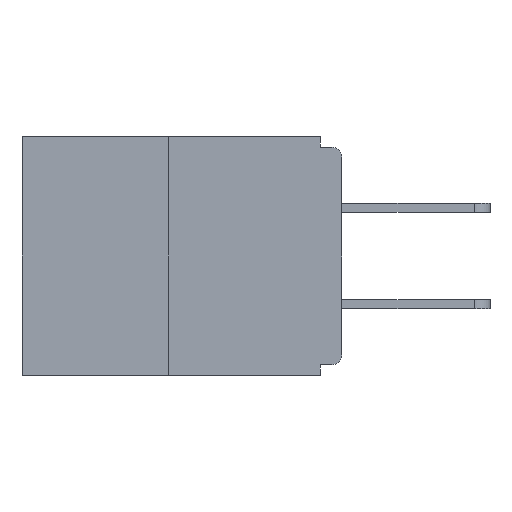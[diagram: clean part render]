
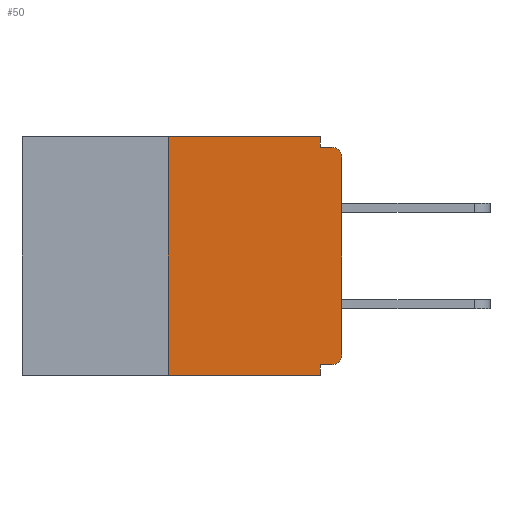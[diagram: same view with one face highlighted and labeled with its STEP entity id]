
A CAD part, left-side view. The second image highlights one B-rep face of the part: STEP entity #50.
In plain terms, the highlighted planar face has unit normal (-1, 0, 0).
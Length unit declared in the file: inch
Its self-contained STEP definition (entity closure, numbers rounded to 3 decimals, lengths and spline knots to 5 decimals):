
#50 = ADVANCED_FACE ( 'NONE', ( #7094 ), #10896, .F. ) ;
#77 = CARTESIAN_POINT ( 'NONE',  ( 0., 0.46, 0. ) ) ;
#176 = VECTOR ( 'NONE', #2043, 39.37008 ) ;
#850 = CARTESIAN_POINT ( 'NONE',  ( 0., 0., -0.313 ) ) ;
#913 = VERTEX_POINT ( 'NONE', #2704 ) ;
#1152 = ORIENTED_EDGE ( 'NONE', *, *, #24956, .F. ) ;
#1242 = EDGE_CURVE ( 'NONE', #12072, #3037, #13367, .T. ) ;
#1349 = VECTOR ( 'NONE', #26919, 39.37008 ) ;
#1949 = DIRECTION ( 'NONE',  ( 0., 0., -1. ) ) ;
#2043 = DIRECTION ( 'NONE',  ( 0., 0., 1. ) ) ;
#2326 = DIRECTION ( 'NONE',  ( 0., 0., -1. ) ) ;
#2608 = CARTESIAN_POINT ( 'NONE',  ( 0., 0.015, -0.015 ) ) ;
#2704 = CARTESIAN_POINT ( 'NONE',  ( 0., 0.25, 0. ) ) ;
#3037 = VERTEX_POINT ( 'NONE', #6431 ) ;
#3648 = CARTESIAN_POINT ( 'NONE',  ( 0., 0.031, -0.343 ) ) ;
#4474 = AXIS2_PLACEMENT_3D ( 'NONE', #77, #15582, #1949 ) ;
#4501 = DIRECTION ( 'NONE',  ( 0., 0., -1. ) ) ;
#4543 = LINE ( 'NONE', #5291, #12303 ) ;
#4746 = EDGE_CURVE ( 'NONE', #8994, #18607, #7180, .T. ) ;
#5291 = CARTESIAN_POINT ( 'NONE',  ( 0., 0.25, 0. ) ) ;
#6322 = EDGE_CURVE ( 'NONE', #14299, #17788, #25975, .T. ) ;
#6391 = DIRECTION ( 'NONE',  ( 0., 1., 0. ) ) ;
#6431 = CARTESIAN_POINT ( 'NONE',  ( 0., 0.031, -0.015 ) ) ;
#6466 = CARTESIAN_POINT ( 'NONE',  ( 0., 0., 0. ) ) ;
#7094 = FACE_OUTER_BOUND ( 'NONE', #17642, .T. ) ;
#7180 = CIRCLE ( 'NONE', #11939, 0.015 ) ;
#7212 = AXIS2_PLACEMENT_3D ( 'NONE', #17928, #15778, #2326 ) ;
#7438 = CARTESIAN_POINT ( 'NONE',  ( 0., 0.031, -0.328 ) ) ;
#8249 = LINE ( 'NONE', #6466, #176 ) ;
#8518 = ORIENTED_EDGE ( 'NONE', *, *, #13809, .F. ) ;
#8994 = VERTEX_POINT ( 'NONE', #19756 ) ;
#9407 = ORIENTED_EDGE ( 'NONE', *, *, #1242, .F. ) ;
#9885 = ORIENTED_EDGE ( 'NONE', *, *, #23658, .T. ) ;
#10427 = DIRECTION ( 'NONE',  ( 0., 0., -1. ) ) ;
#10634 = DIRECTION ( 'NONE',  ( 0., -1., 0. ) ) ;
#10638 = ORIENTED_EDGE ( 'NONE', *, *, #28014, .F. ) ;
#10896 = PLANE ( 'NONE',  #4474 ) ;
#11002 = DIRECTION ( 'NONE',  ( 0., 0., -1. ) ) ;
#11188 = VECTOR ( 'NONE', #28402, 39.37008 ) ;
#11224 = CARTESIAN_POINT ( 'NONE',  ( 0., 0., -0.328 ) ) ;
#11676 = CARTESIAN_POINT ( 'NONE',  ( 0., 0.031, 0. ) ) ;
#11908 = CARTESIAN_POINT ( 'NONE',  ( 0., 0.46, 0. ) ) ;
#11939 = AXIS2_PLACEMENT_3D ( 'NONE', #17849, #22445, #4501 ) ;
#12072 = VERTEX_POINT ( 'NONE', #11676 ) ;
#12303 = VECTOR ( 'NONE', #23337, 39.37008 ) ;
#13057 = CARTESIAN_POINT ( 'NONE',  ( 0., 0., -0.015 ) ) ;
#13367 = LINE ( 'NONE', #24430, #16182 ) ;
#13447 = CARTESIAN_POINT ( 'NONE',  ( 0., 0.46, -0.343 ) ) ;
#13809 = EDGE_CURVE ( 'NONE', #913, #12072, #18185, .T. ) ;
#14072 = ORIENTED_EDGE ( 'NONE', *, *, #15315, .T. ) ;
#14299 = VERTEX_POINT ( 'NONE', #7438 ) ;
#15315 = EDGE_CURVE ( 'NONE', #21755, #8994, #8249, .T. ) ;
#15582 = DIRECTION ( 'NONE',  ( 1., 0., 0. ) ) ;
#15639 = LINE ( 'NONE', #13057, #23108 ) ;
#15778 = DIRECTION ( 'NONE',  ( -1., 0., 0. ) ) ;
#16041 = VECTOR ( 'NONE', #10427, 39.37008 ) ;
#16182 = VECTOR ( 'NONE', #11002, 39.37008 ) ;
#16376 = ORIENTED_EDGE ( 'NONE', *, *, #24390, .F. ) ;
#16398 = EDGE_CURVE ( 'NONE', #28874, #21755, #23719, .T. ) ;
#17642 = EDGE_LOOP ( 'NONE', ( #8518, #10638, #9885, #19010, #16376, #19483, #14072, #22513, #1152, #9407 ) ) ;
#17729 = CARTESIAN_POINT ( 'NONE',  ( 0., 0.031, -0.343 ) ) ;
#17788 = VERTEX_POINT ( 'NONE', #17729 ) ;
#17849 = CARTESIAN_POINT ( 'NONE',  ( 0., 0.015, -0.03 ) ) ;
#17928 = CARTESIAN_POINT ( 'NONE',  ( 0., 0.015, -0.313 ) ) ;
#18185 = LINE ( 'NONE', #11908, #11188 ) ;
#18607 = VERTEX_POINT ( 'NONE', #2608 ) ;
#19010 = ORIENTED_EDGE ( 'NONE', *, *, #6322, .F. ) ;
#19261 = LINE ( 'NONE', #13447, #1349 ) ;
#19483 = ORIENTED_EDGE ( 'NONE', *, *, #16398, .T. ) ;
#19606 = VECTOR ( 'NONE', #6391, 39.37008 ) ;
#19756 = CARTESIAN_POINT ( 'NONE',  ( 0., 0., -0.03 ) ) ;
#20565 = CARTESIAN_POINT ( 'NONE',  ( 0., 0.015, -0.328 ) ) ;
#21755 = VERTEX_POINT ( 'NONE', #850 ) ;
#22149 = LINE ( 'NONE', #11224, #19606 ) ;
#22445 = DIRECTION ( 'NONE',  ( -1., 0., 0. ) ) ;
#22513 = ORIENTED_EDGE ( 'NONE', *, *, #4746, .T. ) ;
#23108 = VECTOR ( 'NONE', #10634, 39.37008 ) ;
#23337 = DIRECTION ( 'NONE',  ( 0., 0., 1. ) ) ;
#23658 = EDGE_CURVE ( 'NONE', #24247, #17788, #19261, .T. ) ;
#23719 = CIRCLE ( 'NONE', #7212, 0.015 ) ;
#24247 = VERTEX_POINT ( 'NONE', #25994 ) ;
#24390 = EDGE_CURVE ( 'NONE', #28874, #14299, #22149, .T. ) ;
#24430 = CARTESIAN_POINT ( 'NONE',  ( 0., 0.031, 0. ) ) ;
#24956 = EDGE_CURVE ( 'NONE', #3037, #18607, #15639, .T. ) ;
#25975 = LINE ( 'NONE', #3648, #16041 ) ;
#25994 = CARTESIAN_POINT ( 'NONE',  ( 0., 0.25, -0.343 ) ) ;
#26919 = DIRECTION ( 'NONE',  ( 0., -1., 0. ) ) ;
#28014 = EDGE_CURVE ( 'NONE', #24247, #913, #4543, .T. ) ;
#28402 = DIRECTION ( 'NONE',  ( 0., -1., 0. ) ) ;
#28874 = VERTEX_POINT ( 'NONE', #20565 ) ;
